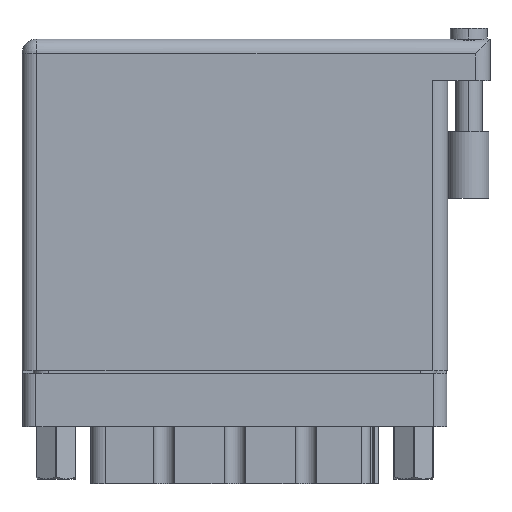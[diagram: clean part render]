
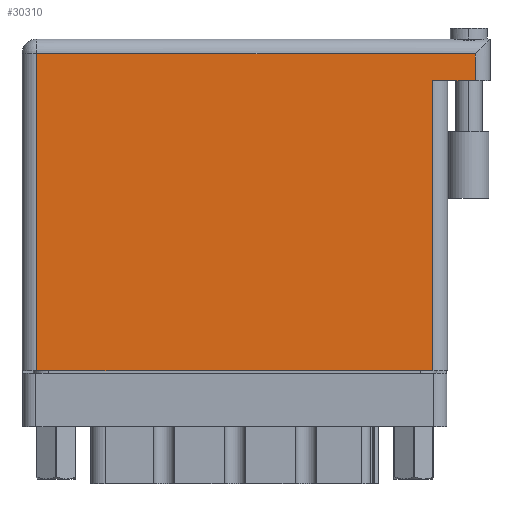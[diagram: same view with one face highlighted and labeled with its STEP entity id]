
A CAD part, front view. The second image highlights one B-rep face of the part: STEP entity #30310.
In plain terms, the highlighted face is planar.
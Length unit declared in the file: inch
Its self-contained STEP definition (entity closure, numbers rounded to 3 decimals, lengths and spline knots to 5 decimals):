
#239 = ORIENTED_EDGE ( 'NONE', *, *, #9261, .T. ) ;
#904 = LINE ( 'NONE', #9416, #26645 ) ;
#1247 = FACE_OUTER_BOUND ( 'NONE', #40871, .T. ) ;
#2423 = DIRECTION ( 'NONE',  ( 0., 0., -1. ) ) ;
#2712 = CARTESIAN_POINT ( 'NONE',  ( 0., 0., 0. ) ) ;
#4191 = CARTESIAN_POINT ( 'NONE',  ( 2.138, 1.369, 0. ) ) ;
#6282 = DIRECTION ( 'NONE',  ( -1., 0., 0. ) ) ;
#6450 = ORIENTED_EDGE ( 'NONE', *, *, #21385, .T. ) ;
#6909 = VECTOR ( 'NONE', #10719, 39.37008 ) ;
#7642 = AXIS2_PLACEMENT_3D ( 'NONE', #21708, #2423, #6282 ) ;
#7648 = VECTOR ( 'NONE', #10298, 39.37008 ) ;
#8109 = CARTESIAN_POINT ( 'NONE',  ( 0.07, 1.496, 0. ) ) ;
#8583 = ORIENTED_EDGE ( 'NONE', *, *, #9466, .F. ) ;
#9261 = EDGE_CURVE ( 'NONE', #15747, #37593, #45194, .T. ) ;
#9416 = CARTESIAN_POINT ( 'NONE',  ( 2.138, 1.566, 0. ) ) ;
#9466 = EDGE_CURVE ( 'NONE', #15200, #37593, #23104, .T. ) ;
#9610 = ORIENTED_EDGE ( 'NONE', *, *, #25040, .T. ) ;
#10298 = DIRECTION ( 'NONE',  ( -1., 0., 0. ) ) ;
#10676 = VERTEX_POINT ( 'NONE', #8109 ) ;
#10719 = DIRECTION ( 'NONE',  ( 0., 1., 0. ) ) ;
#12898 = VECTOR ( 'NONE', #40505, 39.37008 ) ;
#13017 = VECTOR ( 'NONE', #48560, 39.37008 ) ;
#13522 = LINE ( 'NONE', #45166, #20085 ) ;
#13615 = CARTESIAN_POINT ( 'NONE',  ( 2.138, 1.496, 0. ) ) ;
#15200 = VERTEX_POINT ( 'NONE', #4191 ) ;
#15746 = VERTEX_POINT ( 'NONE', #36534 ) ;
#15747 = VERTEX_POINT ( 'NONE', #21355 ) ;
#17200 = ORIENTED_EDGE ( 'NONE', *, *, #37765, .T. ) ;
#17409 = CARTESIAN_POINT ( 'NONE',  ( 2.208, 1.369, 0. ) ) ;
#17660 = PLANE ( 'NONE',  #7642 ) ;
#17838 = LINE ( 'NONE', #2712, #13017 ) ;
#20085 = VECTOR ( 'NONE', #29294, 39.37008 ) ;
#20119 = CARTESIAN_POINT ( 'NONE',  ( 1.938, 1.369, 0. ) ) ;
#21355 = CARTESIAN_POINT ( 'NONE',  ( 1.938, 0., 0. ) ) ;
#21385 = EDGE_CURVE ( 'NONE', #44367, #10676, #38185, .T. ) ;
#21708 = CARTESIAN_POINT ( 'NONE',  ( 0., 1.566, 0. ) ) ;
#23104 = LINE ( 'NONE', #17409, #12898 ) ;
#24231 = CARTESIAN_POINT ( 'NONE',  ( 0., 1.496, 0. ) ) ;
#25040 = EDGE_CURVE ( 'NONE', #15746, #15747, #17838, .T. ) ;
#25457 = CARTESIAN_POINT ( 'NONE',  ( 1.938, 1.369, 0. ) ) ;
#26645 = VECTOR ( 'NONE', #32148, 39.37008 ) ;
#29294 = DIRECTION ( 'NONE',  ( 0., -1., 0. ) ) ;
#30310 = ADVANCED_FACE ( 'NONE', ( #1247 ), #17660, .F. ) ;
#32148 = DIRECTION ( 'NONE',  ( 0., 1., 0. ) ) ;
#33627 = ORIENTED_EDGE ( 'NONE', *, *, #37829, .T. ) ;
#36534 = CARTESIAN_POINT ( 'NONE',  ( 0.07, 0., 0. ) ) ;
#37593 = VERTEX_POINT ( 'NONE', #20119 ) ;
#37765 = EDGE_CURVE ( 'NONE', #15200, #44367, #904, .T. ) ;
#37829 = EDGE_CURVE ( 'NONE', #10676, #15746, #13522, .T. ) ;
#38185 = LINE ( 'NONE', #24231, #7648 ) ;
#40505 = DIRECTION ( 'NONE',  ( -1., 0., 0. ) ) ;
#40871 = EDGE_LOOP ( 'NONE', ( #9610, #239, #8583, #17200, #6450, #33627 ) ) ;
#44367 = VERTEX_POINT ( 'NONE', #13615 ) ;
#45166 = CARTESIAN_POINT ( 'NONE',  ( 0.07, 0., 0. ) ) ;
#45194 = LINE ( 'NONE', #25457, #6909 ) ;
#48560 = DIRECTION ( 'NONE',  ( 1., 0., 0. ) ) ;
